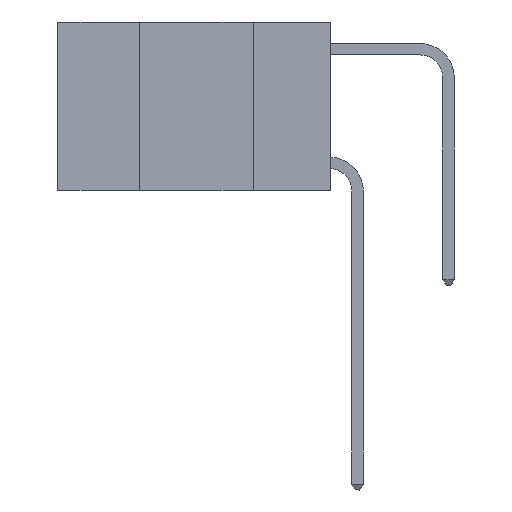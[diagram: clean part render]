
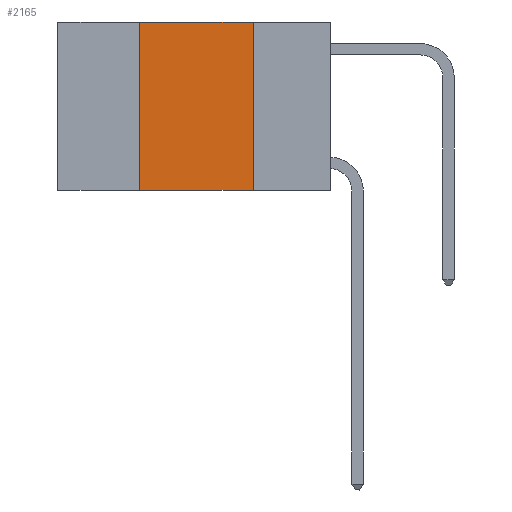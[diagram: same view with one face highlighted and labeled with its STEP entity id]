
A CAD part, left-side view. The second image highlights one B-rep face of the part: STEP entity #2165.
In plain terms, the highlighted planar face has unit normal (-1, 0, 0).
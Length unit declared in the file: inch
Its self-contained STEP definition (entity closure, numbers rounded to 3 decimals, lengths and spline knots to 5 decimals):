
#474 = EDGE_CURVE ( 'NONE', #20049, #10272, #643, .T. ) ;
#643 = LINE ( 'NONE', #5979, #6957 ) ;
#976 = VECTOR ( 'NONE', #18878, 39.37008 ) ;
#1406 = CARTESIAN_POINT ( 'NONE',  ( 0., 0.42, -0.37 ) ) ;
#1695 = DIRECTION ( 'NONE',  ( 1., 0., 0. ) ) ;
#2165 = ADVANCED_FACE ( 'NONE', ( #25342 ), #7733, .F. ) ;
#4129 = ORIENTED_EDGE ( 'NONE', *, *, #20256, .F. ) ;
#4720 = CARTESIAN_POINT ( 'NONE',  ( 0., 0.17, 0. ) ) ;
#4808 = CARTESIAN_POINT ( 'NONE',  ( 0., 0.6, 0. ) ) ;
#5709 = LINE ( 'NONE', #4808, #976 ) ;
#5723 = DIRECTION ( 'NONE',  ( 0., -1., 0. ) ) ;
#5753 = LINE ( 'NONE', #13752, #11725 ) ;
#5979 = CARTESIAN_POINT ( 'NONE',  ( 0., 0.17, 0. ) ) ;
#6957 = VECTOR ( 'NONE', #12047, 39.37008 ) ;
#7566 = DIRECTION ( 'NONE',  ( 0., 0., -1. ) ) ;
#7733 = PLANE ( 'NONE',  #23880 ) ;
#9521 = DIRECTION ( 'NONE',  ( 0., 0., 1. ) ) ;
#10117 = ORIENTED_EDGE ( 'NONE', *, *, #19000, .T. ) ;
#10272 = VERTEX_POINT ( 'NONE', #10956 ) ;
#10956 = CARTESIAN_POINT ( 'NONE',  ( 0., 0.17, -0.37 ) ) ;
#11461 = CARTESIAN_POINT ( 'NONE',  ( 0., 0.42, 0. ) ) ;
#11725 = VECTOR ( 'NONE', #9521, 39.37008 ) ;
#12047 = DIRECTION ( 'NONE',  ( 0., 0., -1. ) ) ;
#13582 = ORIENTED_EDGE ( 'NONE', *, *, #474, .F. ) ;
#13752 = CARTESIAN_POINT ( 'NONE',  ( 0., 0.42, 0. ) ) ;
#13813 = CARTESIAN_POINT ( 'NONE',  ( 0., 0.6, 0. ) ) ;
#14319 = VECTOR ( 'NONE', #5723, 39.37008 ) ;
#14533 = VERTEX_POINT ( 'NONE', #11461 ) ;
#18878 = DIRECTION ( 'NONE',  ( 0., -1., 0. ) ) ;
#19000 = EDGE_CURVE ( 'NONE', #19534, #10272, #19663, .T. ) ;
#19534 = VERTEX_POINT ( 'NONE', #1406 ) ;
#19663 = LINE ( 'NONE', #21615, #14319 ) ;
#20049 = VERTEX_POINT ( 'NONE', #4720 ) ;
#20256 = EDGE_CURVE ( 'NONE', #19534, #14533, #5753, .T. ) ;
#21615 = CARTESIAN_POINT ( 'NONE',  ( 0., 0.6, -0.37 ) ) ;
#22087 = EDGE_LOOP ( 'NONE', ( #13582, #22873, #4129, #10117 ) ) ;
#22873 = ORIENTED_EDGE ( 'NONE', *, *, #23711, .F. ) ;
#23711 = EDGE_CURVE ( 'NONE', #14533, #20049, #5709, .T. ) ;
#23880 = AXIS2_PLACEMENT_3D ( 'NONE', #13813, #1695, #7566 ) ;
#25342 = FACE_OUTER_BOUND ( 'NONE', #22087, .T. ) ;
